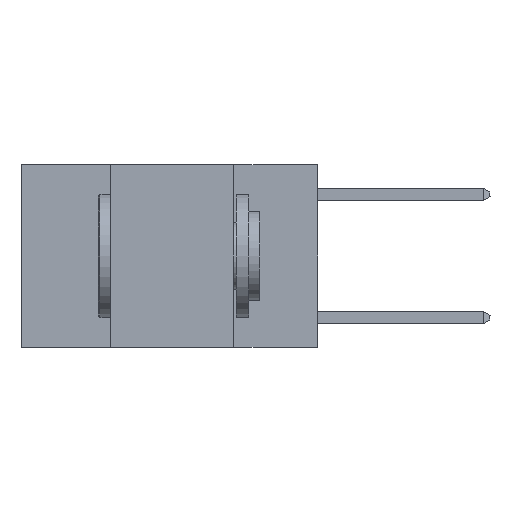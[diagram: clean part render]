
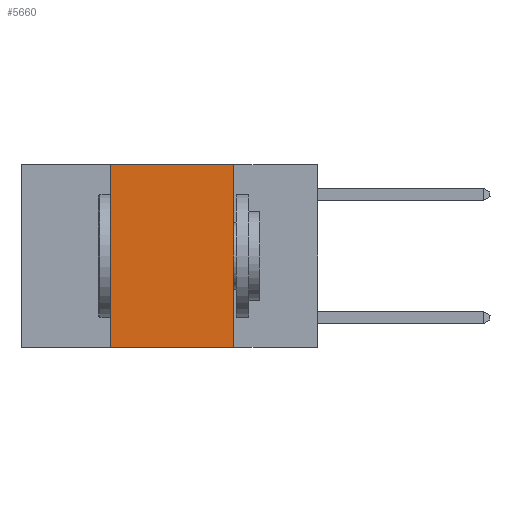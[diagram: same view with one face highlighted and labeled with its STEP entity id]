
A CAD part, left-side view. The second image highlights one B-rep face of the part: STEP entity #5660.
In plain terms, the highlighted planar face has unit normal (-1, 0, 0).
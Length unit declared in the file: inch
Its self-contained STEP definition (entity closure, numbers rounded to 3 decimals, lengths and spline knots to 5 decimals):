
#159 = ORIENTED_EDGE ( 'NONE', *, *, #11146, .F. ) ;
#278 = FACE_OUTER_BOUND ( 'NONE', #10964, .T. ) ;
#704 = VERTEX_POINT ( 'NONE', #5676 ) ;
#1837 = CARTESIAN_POINT ( 'NONE',  ( 0., 0.17, 0. ) ) ;
#2168 = DIRECTION ( 'NONE',  ( 0., 0., 1. ) ) ;
#3180 = EDGE_CURVE ( 'NONE', #704, #14253, #5450, .T. ) ;
#4531 = CARTESIAN_POINT ( 'NONE',  ( 0., 0.42, 0. ) ) ;
#4841 = LINE ( 'NONE', #4992, #14395 ) ;
#4992 = CARTESIAN_POINT ( 'NONE',  ( 0., 0.6, 0. ) ) ;
#5061 = AXIS2_PLACEMENT_3D ( 'NONE', #8221, #13927, #9181 ) ;
#5437 = DIRECTION ( 'NONE',  ( 0., 0., -1. ) ) ;
#5450 = LINE ( 'NONE', #4531, #10767 ) ;
#5660 = ADVANCED_FACE ( 'NONE', ( #278 ), #9331, .F. ) ;
#5676 = CARTESIAN_POINT ( 'NONE',  ( 0., 0.42, -0.37 ) ) ;
#6702 = VERTEX_POINT ( 'NONE', #14510 ) ;
#7688 = EDGE_CURVE ( 'NONE', #704, #6702, #12251, .T. ) ;
#7778 = ORIENTED_EDGE ( 'NONE', *, *, #3180, .F. ) ;
#7797 = CARTESIAN_POINT ( 'NONE',  ( 0., 0.17, 0. ) ) ;
#7950 = CARTESIAN_POINT ( 'NONE',  ( 0., 0.42, 0. ) ) ;
#8013 = CARTESIAN_POINT ( 'NONE',  ( 0., 0.6, -0.37 ) ) ;
#8221 = CARTESIAN_POINT ( 'NONE',  ( 0., 0.6, 0. ) ) ;
#8565 = ORIENTED_EDGE ( 'NONE', *, *, #7688, .T. ) ;
#8785 = ORIENTED_EDGE ( 'NONE', *, *, #10053, .F. ) ;
#8838 = LINE ( 'NONE', #7797, #14155 ) ;
#9181 = DIRECTION ( 'NONE',  ( 0., 0., -1. ) ) ;
#9331 = PLANE ( 'NONE',  #5061 ) ;
#9588 = DIRECTION ( 'NONE',  ( 0., -1., 0. ) ) ;
#10053 = EDGE_CURVE ( 'NONE', #14253, #10598, #4841, .T. ) ;
#10598 = VERTEX_POINT ( 'NONE', #1837 ) ;
#10767 = VECTOR ( 'NONE', #2168, 39.37008 ) ;
#10964 = EDGE_LOOP ( 'NONE', ( #159, #8785, #7778, #8565 ) ) ;
#11146 = EDGE_CURVE ( 'NONE', #10598, #6702, #8838, .T. ) ;
#12251 = LINE ( 'NONE', #8013, #13863 ) ;
#13650 = DIRECTION ( 'NONE',  ( 0., -1., 0. ) ) ;
#13863 = VECTOR ( 'NONE', #13650, 39.37008 ) ;
#13927 = DIRECTION ( 'NONE',  ( 1., 0., 0. ) ) ;
#14155 = VECTOR ( 'NONE', #5437, 39.37008 ) ;
#14253 = VERTEX_POINT ( 'NONE', #7950 ) ;
#14395 = VECTOR ( 'NONE', #9588, 39.37008 ) ;
#14510 = CARTESIAN_POINT ( 'NONE',  ( 0., 0.17, -0.37 ) ) ;
